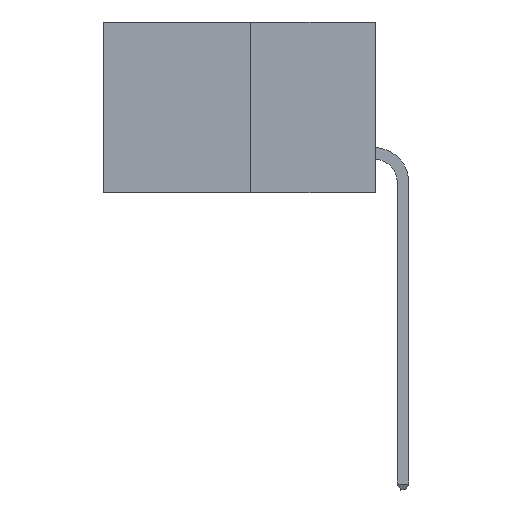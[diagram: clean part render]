
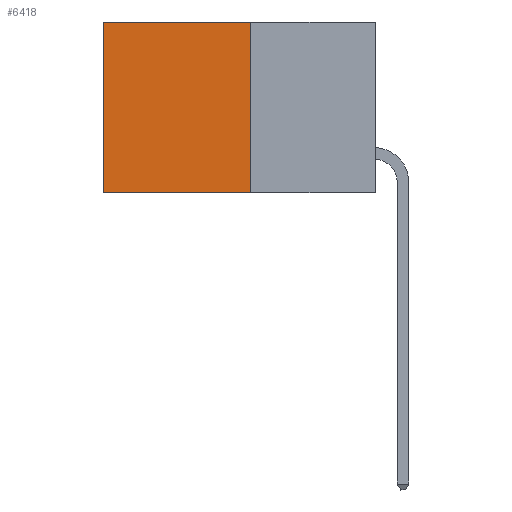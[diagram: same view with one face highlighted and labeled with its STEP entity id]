
A CAD part, left-side view. The second image highlights one B-rep face of the part: STEP entity #6418.
In plain terms, the highlighted planar face has unit normal (-1, 0, 0).
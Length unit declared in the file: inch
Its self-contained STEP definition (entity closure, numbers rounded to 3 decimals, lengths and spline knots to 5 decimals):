
#401 = VERTEX_POINT ( 'NONE', #10656 ) ;
#721 = EDGE_CURVE ( 'NONE', #11463, #401, #4057, .T. ) ;
#920 = CARTESIAN_POINT ( 'NONE',  ( 0.277, 0.27, 0. ) ) ;
#1522 = DIRECTION ( 'NONE',  ( 0., 0., -1. ) ) ;
#1739 = EDGE_CURVE ( 'NONE', #8640, #2681, #6053, .T. ) ;
#1845 = FACE_OUTER_BOUND ( 'NONE', #6559, .T. ) ;
#2273 = ORIENTED_EDGE ( 'NONE', *, *, #10385, .T. ) ;
#2681 = VERTEX_POINT ( 'NONE', #5765 ) ;
#2778 = CARTESIAN_POINT ( 'NONE',  ( 0.277, 0.27, -0.37 ) ) ;
#2874 = DIRECTION ( 'NONE',  ( 0., 1., 0. ) ) ;
#2875 = EDGE_CURVE ( 'NONE', #11463, #8640, #5599, .T. ) ;
#2891 = ORIENTED_EDGE ( 'NONE', *, *, #1739, .F. ) ;
#2896 = DIRECTION ( 'NONE',  ( 0., 0., -1. ) ) ;
#2990 = CARTESIAN_POINT ( 'NONE',  ( 0.277, 0.27, -0.37 ) ) ;
#3113 = ORIENTED_EDGE ( 'NONE', *, *, #2875, .F. ) ;
#3427 = ORIENTED_EDGE ( 'NONE', *, *, #721, .T. ) ;
#4057 = LINE ( 'NONE', #9699, #9806 ) ;
#4233 = AXIS2_PLACEMENT_3D ( 'NONE', #5397, #5174, #5169 ) ;
#5169 = DIRECTION ( 'NONE',  ( 0., 0., -1. ) ) ;
#5174 = DIRECTION ( 'NONE',  ( 1., 0., 0. ) ) ;
#5397 = CARTESIAN_POINT ( 'NONE',  ( 0.277, 0.27, -0.37 ) ) ;
#5409 = CARTESIAN_POINT ( 'NONE',  ( 0.277, 0.59, -0.37 ) ) ;
#5599 = LINE ( 'NONE', #2778, #8098 ) ;
#5626 = VECTOR ( 'NONE', #1522, 39.37008 ) ;
#5692 = PLANE ( 'NONE',  #4233 ) ;
#5765 = CARTESIAN_POINT ( 'NONE',  ( 0.277, 0.59, -0.37 ) ) ;
#5772 = VECTOR ( 'NONE', #2874, 39.37008 ) ;
#6053 = LINE ( 'NONE', #2990, #5772 ) ;
#6418 = ADVANCED_FACE ( 'NONE', ( #1845 ), #5692, .F. ) ;
#6559 = EDGE_LOOP ( 'NONE', ( #2273, #2891, #3113, #3427 ) ) ;
#8098 = VECTOR ( 'NONE', #2896, 39.37008 ) ;
#8446 = LINE ( 'NONE', #5409, #5626 ) ;
#8640 = VERTEX_POINT ( 'NONE', #8683 ) ;
#8683 = CARTESIAN_POINT ( 'NONE',  ( 0.277, 0.27, -0.37 ) ) ;
#9521 = DIRECTION ( 'NONE',  ( 0., 1., 0. ) ) ;
#9699 = CARTESIAN_POINT ( 'NONE',  ( 0.277, 0.27, 0. ) ) ;
#9806 = VECTOR ( 'NONE', #9521, 39.37008 ) ;
#10385 = EDGE_CURVE ( 'NONE', #401, #2681, #8446, .T. ) ;
#10656 = CARTESIAN_POINT ( 'NONE',  ( 0.277, 0.59, 0. ) ) ;
#11463 = VERTEX_POINT ( 'NONE', #920 ) ;
